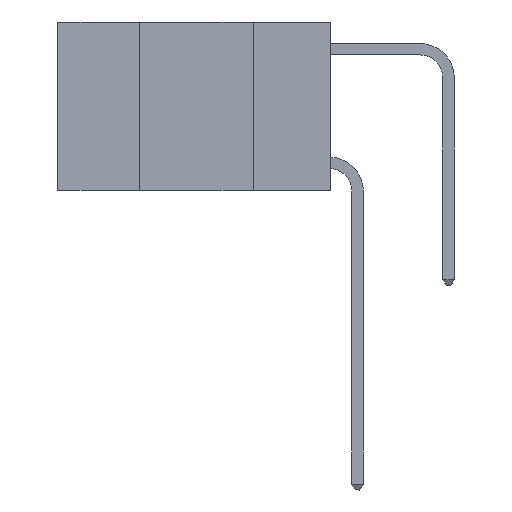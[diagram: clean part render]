
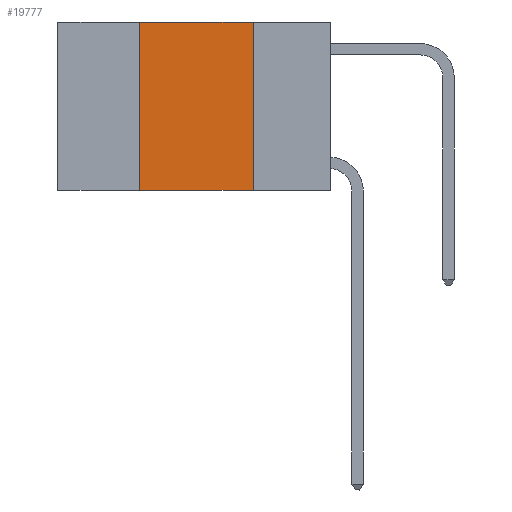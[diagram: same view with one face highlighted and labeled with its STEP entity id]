
A CAD part, left-side view. The second image highlights one B-rep face of the part: STEP entity #19777.
In plain terms, the highlighted planar face has unit normal (-1, 0, 0).
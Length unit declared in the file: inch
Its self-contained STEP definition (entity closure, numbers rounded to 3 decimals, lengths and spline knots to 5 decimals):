
#539 = VERTEX_POINT ( 'NONE', #28358 ) ;
#1149 = LINE ( 'NONE', #4744, #19402 ) ;
#2180 = DIRECTION ( 'NONE',  ( 1., 0., 0. ) ) ;
#4744 = CARTESIAN_POINT ( 'NONE',  ( 0., 0.17, 0. ) ) ;
#4810 = PLANE ( 'NONE',  #23746 ) ;
#6124 = EDGE_CURVE ( 'NONE', #28400, #15579, #12601, .T. ) ;
#7005 = EDGE_CURVE ( 'NONE', #15579, #539, #1149, .T. ) ;
#8818 = FACE_OUTER_BOUND ( 'NONE', #29972, .T. ) ;
#9717 = LINE ( 'NONE', #17852, #10102 ) ;
#10102 = VECTOR ( 'NONE', #28570, 39.37008 ) ;
#10212 = DIRECTION ( 'NONE',  ( 0., 0., -1. ) ) ;
#11157 = DIRECTION ( 'NONE',  ( 0., -1., 0. ) ) ;
#11444 = VERTEX_POINT ( 'NONE', #12725 ) ;
#12601 = LINE ( 'NONE', #19385, #16195 ) ;
#12725 = CARTESIAN_POINT ( 'NONE',  ( 0., 0.42, -0.37 ) ) ;
#13446 = EDGE_CURVE ( 'NONE', #11444, #539, #30570, .T. ) ;
#14364 = ORIENTED_EDGE ( 'NONE', *, *, #13446, .T. ) ;
#15227 = CARTESIAN_POINT ( 'NONE',  ( 0., 0.17, 0. ) ) ;
#15579 = VERTEX_POINT ( 'NONE', #15227 ) ;
#16195 = VECTOR ( 'NONE', #32431, 39.37008 ) ;
#16580 = ORIENTED_EDGE ( 'NONE', *, *, #7005, .F. ) ;
#17852 = CARTESIAN_POINT ( 'NONE',  ( 0., 0.42, 0. ) ) ;
#19385 = CARTESIAN_POINT ( 'NONE',  ( 0., 0.6, 0. ) ) ;
#19402 = VECTOR ( 'NONE', #22794, 39.37008 ) ;
#19777 = ADVANCED_FACE ( 'NONE', ( #8818 ), #4810, .F. ) ;
#21550 = CARTESIAN_POINT ( 'NONE',  ( 0., 0.6, -0.37 ) ) ;
#22778 = ORIENTED_EDGE ( 'NONE', *, *, #6124, .F. ) ;
#22794 = DIRECTION ( 'NONE',  ( 0., 0., -1. ) ) ;
#22852 = ORIENTED_EDGE ( 'NONE', *, *, #25777, .F. ) ;
#23635 = CARTESIAN_POINT ( 'NONE',  ( 0., 0.42, 0. ) ) ;
#23746 = AXIS2_PLACEMENT_3D ( 'NONE', #25820, #2180, #10212 ) ;
#25777 = EDGE_CURVE ( 'NONE', #11444, #28400, #9717, .T. ) ;
#25820 = CARTESIAN_POINT ( 'NONE',  ( 0., 0.6, 0. ) ) ;
#26892 = VECTOR ( 'NONE', #11157, 39.37008 ) ;
#28358 = CARTESIAN_POINT ( 'NONE',  ( 0., 0.17, -0.37 ) ) ;
#28400 = VERTEX_POINT ( 'NONE', #23635 ) ;
#28570 = DIRECTION ( 'NONE',  ( 0., 0., 1. ) ) ;
#29972 = EDGE_LOOP ( 'NONE', ( #16580, #22778, #22852, #14364 ) ) ;
#30570 = LINE ( 'NONE', #21550, #26892 ) ;
#32431 = DIRECTION ( 'NONE',  ( 0., -1., 0. ) ) ;
